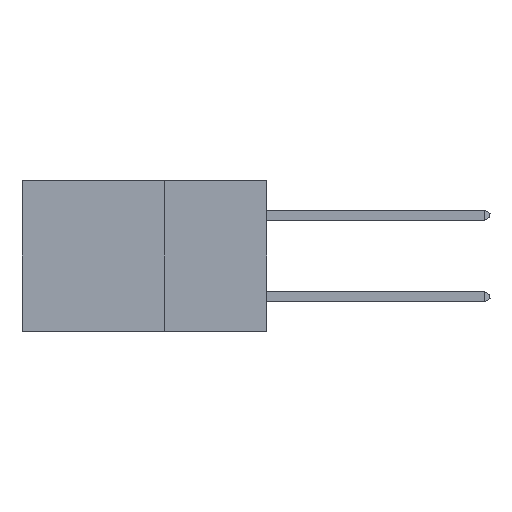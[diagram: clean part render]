
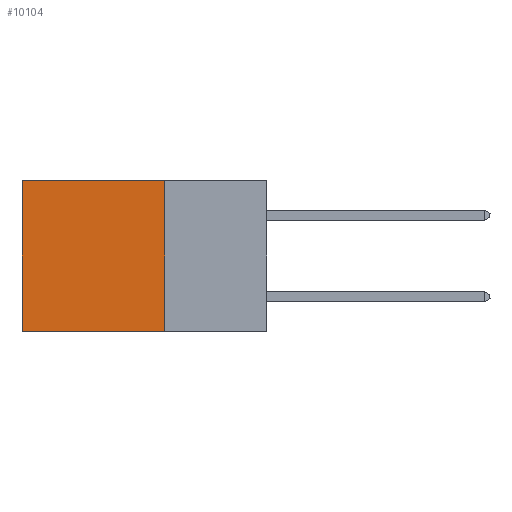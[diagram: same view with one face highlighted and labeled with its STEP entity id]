
A CAD part, left-side view. The second image highlights one B-rep face of the part: STEP entity #10104.
In plain terms, the highlighted planar face has unit normal (-1, 0, 0).
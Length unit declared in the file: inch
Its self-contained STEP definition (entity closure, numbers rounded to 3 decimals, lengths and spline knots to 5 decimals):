
#1321 = DIRECTION ( 'NONE',  ( 0., 0., -1. ) ) ;
#1650 = AXIS2_PLACEMENT_3D ( 'NONE', #10734, #12929, #27486 ) ;
#2296 = CARTESIAN_POINT ( 'NONE',  ( 0.2875, 0.6, -0.37 ) ) ;
#3275 = EDGE_CURVE ( 'NONE', #25647, #15208, #24076, .T. ) ;
#3940 = FACE_OUTER_BOUND ( 'NONE', #19255, .T. ) ;
#4488 = EDGE_CURVE ( 'NONE', #25647, #5946, #26038, .T. ) ;
#5946 = VERTEX_POINT ( 'NONE', #27518 ) ;
#6102 = ORIENTED_EDGE ( 'NONE', *, *, #24118, .T. ) ;
#7060 = VECTOR ( 'NONE', #26544, 39.37008 ) ;
#7290 = DIRECTION ( 'NONE',  ( 0., 1., 0. ) ) ;
#8374 = ORIENTED_EDGE ( 'NONE', *, *, #3275, .F. ) ;
#9148 = CARTESIAN_POINT ( 'NONE',  ( 0.2875, 0.25, -0.37 ) ) ;
#9216 = VECTOR ( 'NONE', #7290, 39.37008 ) ;
#9889 = VECTOR ( 'NONE', #22029, 39.37008 ) ;
#10104 = ADVANCED_FACE ( 'NONE', ( #3940 ), #23401, .F. ) ;
#10382 = CARTESIAN_POINT ( 'NONE',  ( 0.2875, 0.6, 0. ) ) ;
#10734 = CARTESIAN_POINT ( 'NONE',  ( 0.2875, 0.25, 0. ) ) ;
#11381 = CARTESIAN_POINT ( 'NONE',  ( 0.2875, 0.25, -0.37 ) ) ;
#11447 = VECTOR ( 'NONE', #1321, 39.37008 ) ;
#12829 = LINE ( 'NONE', #10382, #11447 ) ;
#12929 = DIRECTION ( 'NONE',  ( 1., 0., 0. ) ) ;
#13349 = VERTEX_POINT ( 'NONE', #2296 ) ;
#15208 = VERTEX_POINT ( 'NONE', #9148 ) ;
#15632 = LINE ( 'NONE', #11381, #9889 ) ;
#19255 = EDGE_LOOP ( 'NONE', ( #6102, #21461, #8374, #22225 ) ) ;
#20265 = CARTESIAN_POINT ( 'NONE',  ( 0.2875, 0.25, 0. ) ) ;
#21338 = EDGE_CURVE ( 'NONE', #15208, #13349, #15632, .T. ) ;
#21461 = ORIENTED_EDGE ( 'NONE', *, *, #21338, .F. ) ;
#22029 = DIRECTION ( 'NONE',  ( 0., 1., 0. ) ) ;
#22225 = ORIENTED_EDGE ( 'NONE', *, *, #4488, .T. ) ;
#23401 = PLANE ( 'NONE',  #1650 ) ;
#23616 = CARTESIAN_POINT ( 'NONE',  ( 0.2875, 0.25, 0. ) ) ;
#24076 = LINE ( 'NONE', #26435, #7060 ) ;
#24118 = EDGE_CURVE ( 'NONE', #5946, #13349, #12829, .T. ) ;
#25647 = VERTEX_POINT ( 'NONE', #23616 ) ;
#26038 = LINE ( 'NONE', #20265, #9216 ) ;
#26435 = CARTESIAN_POINT ( 'NONE',  ( 0.2875, 0.25, 0. ) ) ;
#26544 = DIRECTION ( 'NONE',  ( 0., 0., -1. ) ) ;
#27486 = DIRECTION ( 'NONE',  ( 0., 0., -1. ) ) ;
#27518 = CARTESIAN_POINT ( 'NONE',  ( 0.2875, 0.6, 0. ) ) ;
